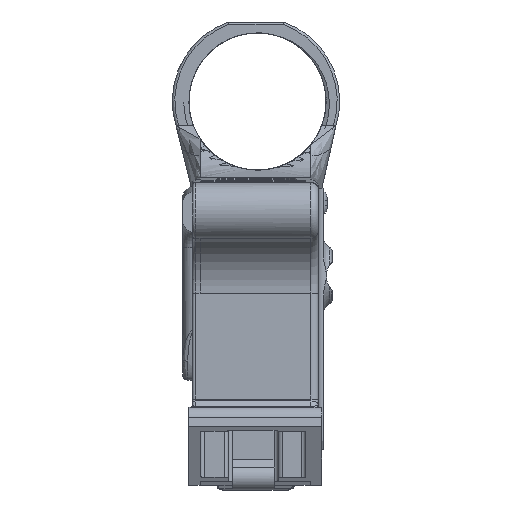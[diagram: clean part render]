
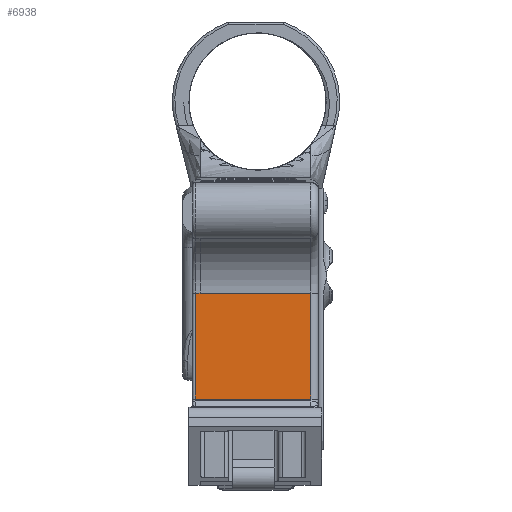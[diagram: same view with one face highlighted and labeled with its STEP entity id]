
A CAD part, left-side view. The second image highlights one B-rep face of the part: STEP entity #6938.
In plain terms, the highlighted planar face has unit normal (-1, 0, 0).
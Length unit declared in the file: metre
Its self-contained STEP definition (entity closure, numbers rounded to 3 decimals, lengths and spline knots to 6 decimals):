
#666=PLANE('',#7671);
#1028=LINE('',#16749,#1453);
#1032=LINE('',#16765,#1457);
#1034=LINE('',#16814,#1459);
#1035=LINE('',#16821,#1460);
#1036=LINE('',#16828,#1461);
#1453=VECTOR('',#9033,1.);
#1457=VECTOR('',#9053,1.);
#1459=VECTOR('',#9085,1.);
#1460=VECTOR('',#9088,1.);
#1461=VECTOR('',#9089,1.);
#2794=ORIENTED_EDGE('',*,*,#4492,.F.);
#2795=ORIENTED_EDGE('',*,*,#4493,.T.);
#2796=ORIENTED_EDGE('',*,*,#4490,.T.);
#2797=ORIENTED_EDGE('',*,*,#4472,.T.);
#2798=ORIENTED_EDGE('',*,*,#4479,.T.);
#2799=ORIENTED_EDGE('',*,*,#4494,.F.);
#4472=EDGE_CURVE('',#5340,#5337,#1028,.T.);
#4479=EDGE_CURVE('',#5337,#5342,#1032,.T.);
#4490=EDGE_CURVE('',#5352,#5340,#1034,.T.);
#4492=EDGE_CURVE('',#5353,#5354,#1035,.T.);
#4493=EDGE_CURVE('',#5353,#5352,#5658,.T.);
#4494=EDGE_CURVE('',#5354,#5342,#1036,.T.);
#5337=VERTEX_POINT('',#16736);
#5340=VERTEX_POINT('',#16746);
#5342=VERTEX_POINT('',#16766);
#5352=VERTEX_POINT('',#16815);
#5353=VERTEX_POINT('',#16822);
#5354=VERTEX_POINT('',#16823);
#5658=B_SPLINE_CURVE_WITH_KNOTS('',3,(#16824,#16825,#16826,#16827),
 .UNSPECIFIED.,.F.,.F.,(4,4),(0.,1.),.UNSPECIFIED.);
#6008=EDGE_LOOP('',(#2794,#2795,#2796,#2797,#2798,#2799));
#6472=FACE_BOUND('',#6008,.T.);
#6938=ADVANCED_FACE('',(#6472),#666,.F.);
#7671=AXIS2_PLACEMENT_3D('',#16820,#9086,#9087);
#9033=DIRECTION('',(0.,0.,1.));
#9053=DIRECTION('',(0.,1.,0.));
#9085=DIRECTION('',(0.,-1.,0.));
#9086=DIRECTION('',(1.,0.,0.));
#9087=DIRECTION('',(0.,0.,-1.));
#9088=DIRECTION('',(0.,-1.,0.));
#9089=DIRECTION('',(0.,-1.,0.));
#16736=CARTESIAN_POINT('',(-0.163693,-0.0761,-0.007442));
#16746=CARTESIAN_POINT('',(-0.163693,-0.0761,-0.049822));
#16749=CARTESIAN_POINT('',(-0.163693,-0.0761,-0.007442));
#16765=CARTESIAN_POINT('',(-0.163693,-0.0791,-0.007442));
#16766=CARTESIAN_POINT('',(-0.163693,-0.076,-0.007442));
#16814=CARTESIAN_POINT('',(-0.163693,-0.0317,-0.049822));
#16815=CARTESIAN_POINT('',(-0.163693,-0.0297,-0.049822));
#16820=CARTESIAN_POINT('',(-0.163693,-0.0317,-0.028632));
#16821=CARTESIAN_POINT('',(-0.163693,-0.0287,-0.007442));
#16822=CARTESIAN_POINT('',(-0.163693,-0.0297,-0.007442));
#16823=CARTESIAN_POINT('',(-0.163693,-0.0317,-0.007442));
#16824=CARTESIAN_POINT('',(-0.163693,-0.0297,-0.007442));
#16825=CARTESIAN_POINT('',(-0.163693,-0.0297,-0.021569));
#16826=CARTESIAN_POINT('',(-0.163693,-0.0297,-0.035695));
#16827=CARTESIAN_POINT('',(-0.163693,-0.0297,-0.049822));
#16828=CARTESIAN_POINT('',(-0.163693,-0.0317,-0.007442));
